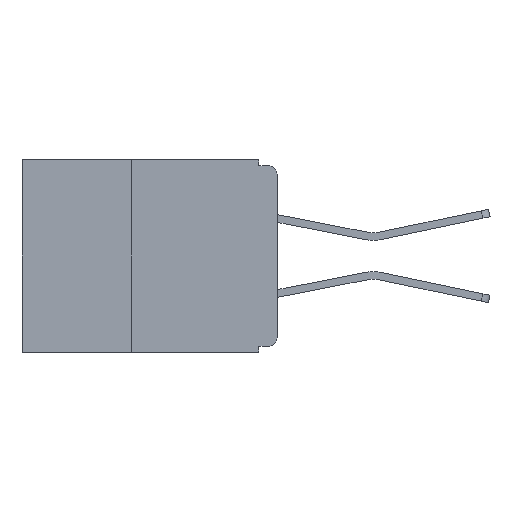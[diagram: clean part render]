
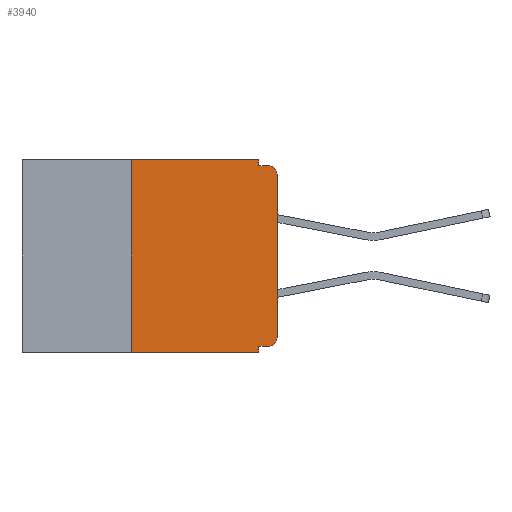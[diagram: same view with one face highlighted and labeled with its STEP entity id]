
A CAD part, left-side view. The second image highlights one B-rep face of the part: STEP entity #3940.
In plain terms, the highlighted planar face has unit normal (-1, 0, 0).
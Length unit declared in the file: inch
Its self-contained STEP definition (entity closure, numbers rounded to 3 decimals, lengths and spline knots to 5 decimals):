
#151 = CARTESIAN_POINT ( 'NONE',  ( 0., 0.25, -0.33 ) ) ;
#689 = CARTESIAN_POINT ( 'NONE',  ( 0., 0., -0.025 ) ) ;
#796 = LINE ( 'NONE', #16714, #5408 ) ;
#1032 = VERTEX_POINT ( 'NONE', #12239 ) ;
#1487 = DIRECTION ( 'NONE',  ( -1., 0., 0. ) ) ;
#1538 = CIRCLE ( 'NONE', #13478, 0.015 ) ;
#1567 = VERTEX_POINT ( 'NONE', #15515 ) ;
#1912 = EDGE_LOOP ( 'NONE', ( #24793, #22139, #23069, #3932, #6386, #5563, #12874, #15976, #8758, #24596 ) ) ;
#2556 = CARTESIAN_POINT ( 'NONE',  ( 0., 0.015, -0.025 ) ) ;
#2642 = LINE ( 'NONE', #7511, #22724 ) ;
#2713 = LINE ( 'NONE', #14875, #13108 ) ;
#3331 = DIRECTION ( 'NONE',  ( 0., 0., -1. ) ) ;
#3558 = VECTOR ( 'NONE', #22435, 39.37008 ) ;
#3789 = CARTESIAN_POINT ( 'NONE',  ( 0., 0.031, -0.33 ) ) ;
#3932 = ORIENTED_EDGE ( 'NONE', *, *, #14031, .F. ) ;
#3940 = ADVANCED_FACE ( 'NONE', ( #15692 ), #9745, .F. ) ;
#4072 = AXIS2_PLACEMENT_3D ( 'NONE', #2556, #16194, #4544 ) ;
#4525 = VECTOR ( 'NONE', #3331, 39.37008 ) ;
#4544 = DIRECTION ( 'NONE',  ( 0., 0., -1. ) ) ;
#5172 = DIRECTION ( 'NONE',  ( 0., 0., 1. ) ) ;
#5408 = VECTOR ( 'NONE', #9493, 39.37008 ) ;
#5563 = ORIENTED_EDGE ( 'NONE', *, *, #12694, .F. ) ;
#5672 = CARTESIAN_POINT ( 'NONE',  ( 0., 0.031, -0.33 ) ) ;
#6386 = ORIENTED_EDGE ( 'NONE', *, *, #19833, .F. ) ;
#7502 = EDGE_CURVE ( 'NONE', #8392, #10115, #9735, .T. ) ;
#7511 = CARTESIAN_POINT ( 'NONE',  ( 0., 0.031, 0. ) ) ;
#8181 = EDGE_CURVE ( 'NONE', #24120, #1567, #24167, .T. ) ;
#8392 = VERTEX_POINT ( 'NONE', #18528 ) ;
#8475 = VECTOR ( 'NONE', #12206, 39.37008 ) ;
#8758 = ORIENTED_EDGE ( 'NONE', *, *, #22967, .F. ) ;
#8815 = EDGE_CURVE ( 'NONE', #15959, #10115, #796, .T. ) ;
#9074 = DIRECTION ( 'NONE',  ( 0., 0., -1. ) ) ;
#9491 = DIRECTION ( 'NONE',  ( 0., 0., -1. ) ) ;
#9493 = DIRECTION ( 'NONE',  ( 0., -1., 0. ) ) ;
#9735 = LINE ( 'NONE', #3789, #4525 ) ;
#9745 = PLANE ( 'NONE',  #18268 ) ;
#10115 = VERTEX_POINT ( 'NONE', #5672 ) ;
#10321 = CARTESIAN_POINT ( 'NONE',  ( 0., 0., 0. ) ) ;
#11456 = DIRECTION ( 'NONE',  ( 1., 0., 0. ) ) ;
#12114 = DIRECTION ( 'NONE',  ( 0., -1., 0. ) ) ;
#12206 = DIRECTION ( 'NONE',  ( 0., 0., 1. ) ) ;
#12239 = CARTESIAN_POINT ( 'NONE',  ( 0., 0.015, -0.32 ) ) ;
#12694 = EDGE_CURVE ( 'NONE', #15959, #16463, #2713, .T. ) ;
#12874 = ORIENTED_EDGE ( 'NONE', *, *, #8815, .T. ) ;
#13108 = VECTOR ( 'NONE', #5172, 39.37008 ) ;
#13194 = CARTESIAN_POINT ( 'NONE',  ( 0., 0.015, -0.305 ) ) ;
#13478 = AXIS2_PLACEMENT_3D ( 'NONE', #13194, #1487, #15147 ) ;
#14031 = EDGE_CURVE ( 'NONE', #18478, #24120, #2642, .T. ) ;
#14494 = VECTOR ( 'NONE', #12114, 39.37008 ) ;
#14875 = CARTESIAN_POINT ( 'NONE',  ( 0., 0.25, -0.33 ) ) ;
#14926 = VECTOR ( 'NONE', #22920, 39.37008 ) ;
#14973 = VERTEX_POINT ( 'NONE', #689 ) ;
#15147 = DIRECTION ( 'NONE',  ( 0., 0., -1. ) ) ;
#15515 = CARTESIAN_POINT ( 'NONE',  ( 0., 0.015, -0.01 ) ) ;
#15661 = CARTESIAN_POINT ( 'NONE',  ( 0., 0.031, 0. ) ) ;
#15692 = FACE_OUTER_BOUND ( 'NONE', #1912, .T. ) ;
#15959 = VERTEX_POINT ( 'NONE', #151 ) ;
#15976 = ORIENTED_EDGE ( 'NONE', *, *, #7502, .F. ) ;
#16194 = DIRECTION ( 'NONE',  ( -1., 0., 0. ) ) ;
#16463 = VERTEX_POINT ( 'NONE', #24643 ) ;
#16476 = EDGE_CURVE ( 'NONE', #1032, #18680, #1538, .T. ) ;
#16714 = CARTESIAN_POINT ( 'NONE',  ( 0., 0.437, -0.33 ) ) ;
#17187 = CIRCLE ( 'NONE', #4072, 0.015 ) ;
#18227 = CARTESIAN_POINT ( 'NONE',  ( 0., 0.437, 0. ) ) ;
#18268 = AXIS2_PLACEMENT_3D ( 'NONE', #18227, #11456, #9074 ) ;
#18478 = VERTEX_POINT ( 'NONE', #15661 ) ;
#18528 = CARTESIAN_POINT ( 'NONE',  ( 0., 0.031, -0.32 ) ) ;
#18634 = EDGE_CURVE ( 'NONE', #18680, #14973, #23900, .T. ) ;
#18680 = VERTEX_POINT ( 'NONE', #23956 ) ;
#19833 = EDGE_CURVE ( 'NONE', #16463, #18478, #20267, .T. ) ;
#20108 = LINE ( 'NONE', #20995, #14926 ) ;
#20267 = LINE ( 'NONE', #23802, #14494 ) ;
#20393 = EDGE_CURVE ( 'NONE', #14973, #1567, #17187, .T. ) ;
#20483 = CARTESIAN_POINT ( 'NONE',  ( 0., 0., -0.01 ) ) ;
#20995 = CARTESIAN_POINT ( 'NONE',  ( 0., 0., -0.32 ) ) ;
#22139 = ORIENTED_EDGE ( 'NONE', *, *, #20393, .T. ) ;
#22435 = DIRECTION ( 'NONE',  ( 0., -1., 0. ) ) ;
#22724 = VECTOR ( 'NONE', #9491, 39.37008 ) ;
#22920 = DIRECTION ( 'NONE',  ( 0., 1., 0. ) ) ;
#22967 = EDGE_CURVE ( 'NONE', #1032, #8392, #20108, .T. ) ;
#23069 = ORIENTED_EDGE ( 'NONE', *, *, #8181, .F. ) ;
#23802 = CARTESIAN_POINT ( 'NONE',  ( 0., 0.437, 0. ) ) ;
#23900 = LINE ( 'NONE', #10321, #8475 ) ;
#23956 = CARTESIAN_POINT ( 'NONE',  ( 0., 0., -0.305 ) ) ;
#24120 = VERTEX_POINT ( 'NONE', #24413 ) ;
#24167 = LINE ( 'NONE', #20483, #3558 ) ;
#24413 = CARTESIAN_POINT ( 'NONE',  ( 0., 0.031, -0.01 ) ) ;
#24596 = ORIENTED_EDGE ( 'NONE', *, *, #16476, .T. ) ;
#24643 = CARTESIAN_POINT ( 'NONE',  ( 0., 0.25, 0. ) ) ;
#24793 = ORIENTED_EDGE ( 'NONE', *, *, #18634, .T. ) ;
